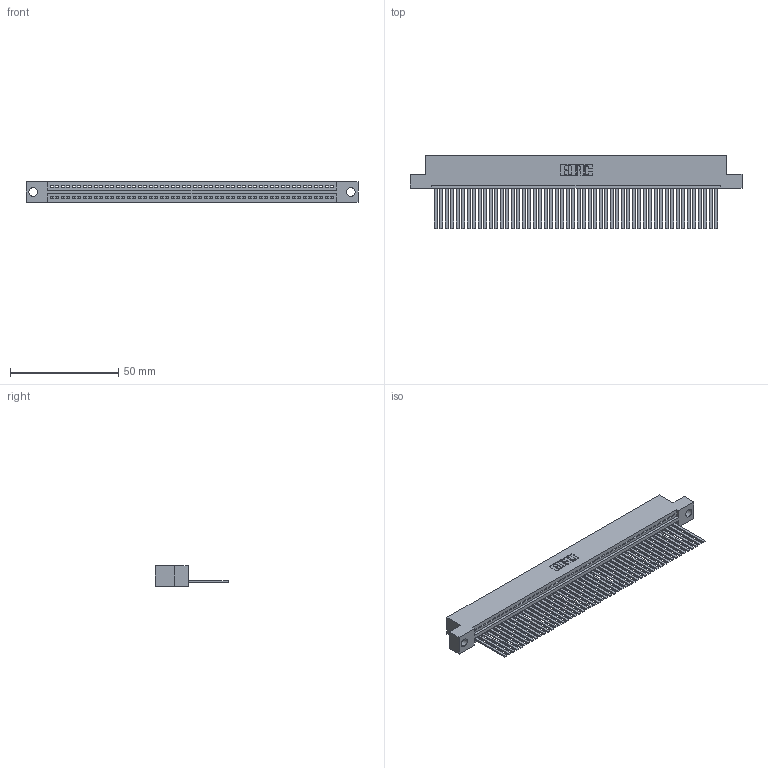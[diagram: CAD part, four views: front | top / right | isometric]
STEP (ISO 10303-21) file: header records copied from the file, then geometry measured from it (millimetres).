
FILE_DESCRIPTION (( 'STEP AP203' ), '1' );
FILE_NAME ('345-052-544-104.STEP', '2019-10-09T19:17:52', ( '' ), ( '' ), 'SwSTEP 2.0', 'SolidWorks 2016', '' );
FILE_SCHEMA (( 'CONFIG_CONTROL_DESIGN' ));
Length unit declared in the file: inch
Products named in the file (3): 345-052-544-104; 345 Part_Flush Mounting Lugs - 0.156 Dia-TH; 345-292-001_345-293-144
Assembly tree (53 placements, depth 2):
  345-052-544-104
    345 Part_Flush Mounting Lugs - 0.156 Dia-TH
    345-292-001_345-293-144  x52
Bounding box: 153.29 x 33.96 x 9.4 mm (x, y, z)
Volume: 15155.8 mm3; surface area: 21893.4 mm2
Topology: 53 solids, 53 shells, 2830 faces, 8557 edges, 5634 vertices
Faces by surface type: plane 1952, cylinder 878
Entity records: 37609 total; most frequent: CARTESIAN_POINT 6520, ORIENTED_EDGE 6506, DIRECTION 5677, EDGE_CURVE 3253, LINE 2917, VECTOR 2917, VERTEX_POINT 2166, AXIS2_PLACEMENT_3D 1380
